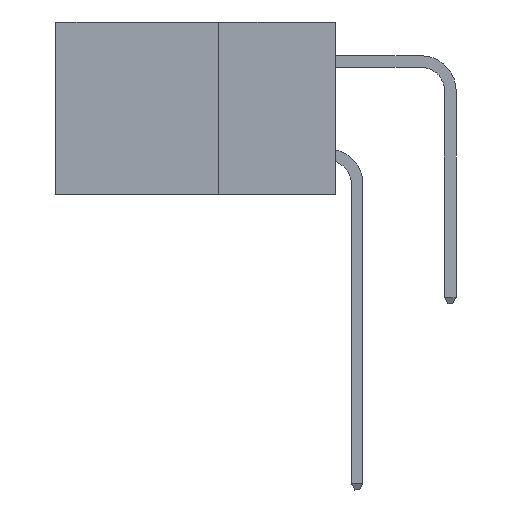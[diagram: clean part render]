
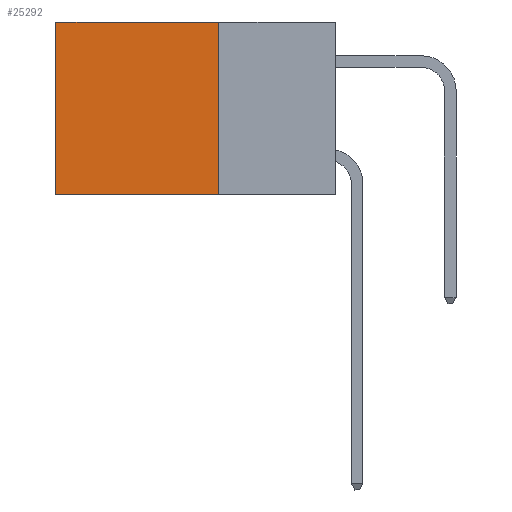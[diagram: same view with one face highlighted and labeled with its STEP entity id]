
A CAD part, left-side view. The second image highlights one B-rep face of the part: STEP entity #25292.
In plain terms, the highlighted planar face has unit normal (-1, 0, 0).
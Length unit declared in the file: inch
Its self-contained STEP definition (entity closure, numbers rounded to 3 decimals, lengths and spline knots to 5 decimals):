
#1190 = PLANE ( 'NONE',  #23406 ) ;
#4347 = CARTESIAN_POINT ( 'NONE',  ( 0.2875, 0.25, 0. ) ) ;
#5233 = DIRECTION ( 'NONE',  ( 0., 0., -1. ) ) ;
#6990 = VERTEX_POINT ( 'NONE', #33413 ) ;
#7143 = EDGE_CURVE ( 'NONE', #6990, #14664, #16839, .T. ) ;
#7955 = EDGE_LOOP ( 'NONE', ( #28380, #15622, #23024, #21813 ) ) ;
#9048 = LINE ( 'NONE', #36394, #25405 ) ;
#11069 = DIRECTION ( 'NONE',  ( 0., 1., 0. ) ) ;
#13887 = VERTEX_POINT ( 'NONE', #30523 ) ;
#14664 = VERTEX_POINT ( 'NONE', #29150 ) ;
#14918 = VERTEX_POINT ( 'NONE', #4347 ) ;
#15622 = ORIENTED_EDGE ( 'NONE', *, *, #21219, .F. ) ;
#16794 = CARTESIAN_POINT ( 'NONE',  ( 0.2875, 0.6, 0. ) ) ;
#16839 = LINE ( 'NONE', #16794, #19103 ) ;
#16903 = CARTESIAN_POINT ( 'NONE',  ( 0.2875, 0.25, -0.37 ) ) ;
#19103 = VECTOR ( 'NONE', #5233, 39.37008 ) ;
#20122 = LINE ( 'NONE', #16903, #26253 ) ;
#20839 = CARTESIAN_POINT ( 'NONE',  ( 0.2875, 0.25, 0. ) ) ;
#21219 = EDGE_CURVE ( 'NONE', #13887, #14664, #20122, .T. ) ;
#21408 = DIRECTION ( 'NONE',  ( 0., 1., 0. ) ) ;
#21813 = ORIENTED_EDGE ( 'NONE', *, *, #34808, .T. ) ;
#23024 = ORIENTED_EDGE ( 'NONE', *, *, #29983, .F. ) ;
#23312 = DIRECTION ( 'NONE',  ( 0., 0., -1. ) ) ;
#23406 = AXIS2_PLACEMENT_3D ( 'NONE', #20839, #35133, #26621 ) ;
#25292 = ADVANCED_FACE ( 'NONE', ( #27354 ), #1190, .F. ) ;
#25405 = VECTOR ( 'NONE', #11069, 39.37008 ) ;
#26253 = VECTOR ( 'NONE', #21408, 39.37008 ) ;
#26621 = DIRECTION ( 'NONE',  ( 0., 0., -1. ) ) ;
#27354 = FACE_OUTER_BOUND ( 'NONE', #7955, .T. ) ;
#28380 = ORIENTED_EDGE ( 'NONE', *, *, #7143, .T. ) ;
#28983 = CARTESIAN_POINT ( 'NONE',  ( 0.2875, 0.25, 0. ) ) ;
#29150 = CARTESIAN_POINT ( 'NONE',  ( 0.2875, 0.6, -0.37 ) ) ;
#29983 = EDGE_CURVE ( 'NONE', #14918, #13887, #30231, .T. ) ;
#30231 = LINE ( 'NONE', #28983, #31102 ) ;
#30523 = CARTESIAN_POINT ( 'NONE',  ( 0.2875, 0.25, -0.37 ) ) ;
#31102 = VECTOR ( 'NONE', #23312, 39.37008 ) ;
#33413 = CARTESIAN_POINT ( 'NONE',  ( 0.2875, 0.6, 0. ) ) ;
#34808 = EDGE_CURVE ( 'NONE', #14918, #6990, #9048, .T. ) ;
#35133 = DIRECTION ( 'NONE',  ( 1., 0., 0. ) ) ;
#36394 = CARTESIAN_POINT ( 'NONE',  ( 0.2875, 0.25, 0. ) ) ;
